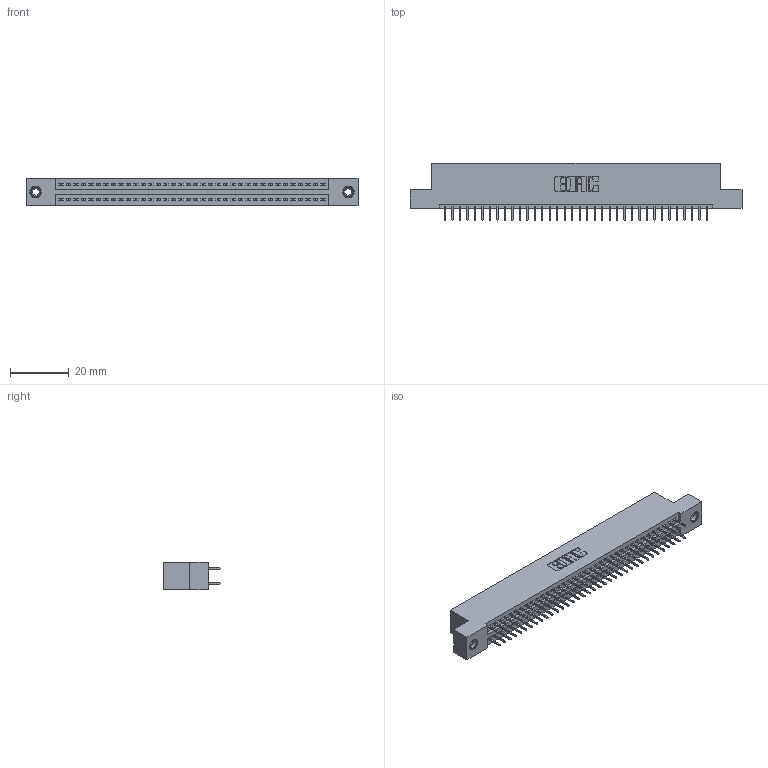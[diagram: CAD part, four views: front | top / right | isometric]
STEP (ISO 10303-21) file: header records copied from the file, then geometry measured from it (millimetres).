
FILE_DESCRIPTION (( 'STEP AP203' ), '1' );
FILE_NAME ('345-072-524-208.STEP', '2018-10-02T05:12:17', ( '' ), ( '' ), 'SwSTEP 2.0', 'SolidWorks 2016', '' );
FILE_SCHEMA (( 'CONFIG_CONTROL_DESIGN' ));
Length unit declared in the file: inch
Products named in the file (4): 345-250-001_345-250-003-102; 345-072-524-208; 345-292-001_345-293-124; 345 Part_Flush Mounting Lugs - 0.156 Dia-TI
Assembly tree (75 placements, depth 2):
  345-072-524-208
    345 Part_Flush Mounting Lugs - 0.156 Dia-TI
    345-292-001_345-293-124  x72
    345-250-001_345-250-003-102  x2
Bounding box: 112.65 x 19.35 x 9.4 mm (x, y, z)
Volume: 10771.7 mm3; surface area: 15531.9 mm2
Topology: 75 solids, 75 shells, 4074 faces, 11493 edges, 7366 vertices
Faces by surface type: plane 2920, cylinder 1138, cone 12, torus 4
Entity records: 30314 total; most frequent: CARTESIAN_POINT 5067, ORIENTED_EDGE 4994, DIRECTION 4503, EDGE_CURVE 2497, LINE 2205, VECTOR 2205, VERTEX_POINT 1656, AXIS2_PLACEMENT_3D 1149
